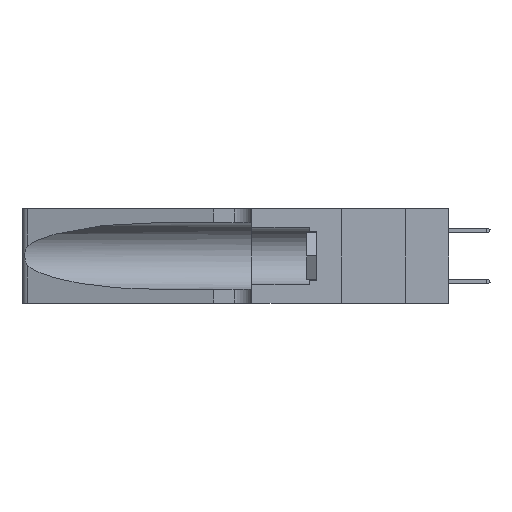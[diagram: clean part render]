
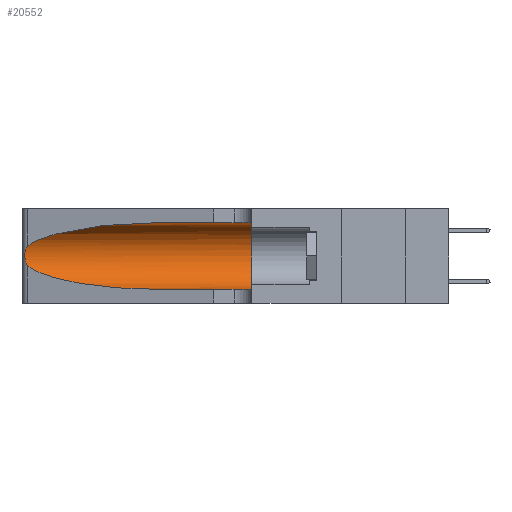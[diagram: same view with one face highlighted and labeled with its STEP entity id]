
A CAD part, left-side view. The second image highlights one B-rep face of the part: STEP entity #20552.
In plain terms, the highlighted cylindrical face has radius 3.308 mm (diameter 6.617 mm), a partial arc.
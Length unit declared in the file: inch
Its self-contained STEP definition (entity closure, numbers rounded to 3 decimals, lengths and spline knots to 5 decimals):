
#764 = EDGE_CURVE ( 'NONE', #38939, #9621, #17891, .T. ) ;
#1037 = CARTESIAN_POINT ( 'NONE',  ( 0.25487, 1.22718, 0.22369 ) ) ;
#1170 = CARTESIAN_POINT ( 'NONE',  ( 0.26075, 1.23896, 0.19203 ) ) ;
#2813 =( BOUNDED_CURVE ( )  B_SPLINE_CURVE ( 3, ( #10790, #7544, #30076, #33336 ),
 .UNSPECIFIED., .F., .F. ) 
 B_SPLINE_CURVE_WITH_KNOTS ( ( 4, 4 ),
 ( 1.5708, 2.84003 ),
 .UNSPECIFIED. ) 
 CURVE ( )  GEOMETRIC_REPRESENTATION_ITEM ( )  RATIONAL_B_SPLINE_CURVE ( ( 1., 0.87, 0.87, 1. ) ) 
 REPRESENTATION_ITEM ( '' )  );
#4483 = CARTESIAN_POINT ( 'NONE',  ( 0.26017, 1.23833, 0.17102 ) ) ;
#5992 = ORIENTED_EDGE ( 'NONE', *, *, #22381, .F. ) ;
#6490 = CARTESIAN_POINT ( 'NONE',  ( 0.25487, 1.22718, 0.14631 ) ) ;
#6668 = EDGE_CURVE ( 'NONE', #27552, #9397, #2813, .T. ) ;
#7430 = CARTESIAN_POINT ( 'NONE',  ( 0.1305, 1.61858, 0.05475 ) ) ;
#7544 = CARTESIAN_POINT ( 'NONE',  ( 0.18966, 0.96281, 0.31525 ) ) ;
#7632 = CARTESIAN_POINT ( 'NONE',  ( 0.25555, 1.22994, 0.2215 ) ) ;
#7770 = CARTESIAN_POINT ( 'NONE',  ( 0.25789, 1.23486, 0.15765 ) ) ;
#8104 = CYLINDRICAL_SURFACE ( 'NONE', #29977, 0.13025 ) ;
#8883 = CARTESIAN_POINT ( 'NONE',  ( 0.1305, 0.35, 0.05475 ) ) ;
#9397 = VERTEX_POINT ( 'NONE', #16761 ) ;
#9621 = VERTEX_POINT ( 'NONE', #17866 ) ;
#10143 = FACE_OUTER_BOUND ( 'NONE', #13462, .T. ) ;
#10790 = CARTESIAN_POINT ( 'NONE',  ( 0.1305, 0.72297, 0.31525 ) ) ;
#11026 = CARTESIAN_POINT ( 'NONE',  ( 0.25555, 1.22993, 0.14849 ) ) ;
#11373 = ORIENTED_EDGE ( 'NONE', *, *, #764, .T. ) ;
#11673 = B_SPLINE_CURVE_WITH_KNOTS ( 'NONE', 3,
 ( #1037, #7632, #36651, #17365, #39866, #20601, #1170, #23839, #4483, #27059, #7770, #30301, #11026, #33558 ),
 .UNSPECIFIED., .F., .F.,
 ( 4, 2, 2, 2, 2, 2, 4 ),
 ( 0., 0.00027, 0.00053, 0.00107, 0.0016, 0.00187, 0.00214 ),
 .UNSPECIFIED. ) ;
#12667 = CARTESIAN_POINT ( 'NONE',  ( 0.1305, 1.61858, 0.185 ) ) ;
#13123 = CARTESIAN_POINT ( 'NONE',  ( 0.1305, 0.35, 0.185 ) ) ;
#13462 = EDGE_LOOP ( 'NONE', ( #30935, #40917, #11373, #40772, #5992, #27935 ) ) ;
#14222 = CARTESIAN_POINT ( 'NONE',  ( 0.2373, 1.15595, 0.08982 ) ) ;
#15902 = DIRECTION ( 'NONE',  ( 0., 0., -1. ) ) ;
#16385 = DIRECTION ( 'NONE',  ( 0., 0., 1. ) ) ;
#16761 = CARTESIAN_POINT ( 'NONE',  ( 0.25487, 1.22718, 0.22369 ) ) ;
#17365 = CARTESIAN_POINT ( 'NONE',  ( 0.25787, 1.23484, 0.2124 ) ) ;
#17489 = CARTESIAN_POINT ( 'NONE',  ( 0.1305, 0.72297, 0.05475 ) ) ;
#17866 = CARTESIAN_POINT ( 'NONE',  ( 0.1305, 0.72297, 0.05475 ) ) ;
#17891 =( BOUNDED_CURVE ( )  B_SPLINE_CURVE ( 3, ( #27045, #14222, #33543, #17489 ),
 .UNSPECIFIED., .F., .T. ) 
 B_SPLINE_CURVE_WITH_KNOTS ( ( 4, 4 ),
 ( 3.44316, 4.71239 ),
 .UNSPECIFIED. ) 
 CURVE ( )  GEOMETRIC_REPRESENTATION_ITEM ( )  RATIONAL_B_SPLINE_CURVE ( ( 1., 0.87, 0.87, 1. ) ) 
 REPRESENTATION_ITEM ( '' )  );
#18500 = CARTESIAN_POINT ( 'NONE',  ( 0.1305, 1.61858, 0.31525 ) ) ;
#19643 = LINE ( 'NONE', #18500, #35775 ) ;
#20552 = ADVANCED_FACE ( 'NONE', ( #10143 ), #8104, .F. ) ;
#20601 = CARTESIAN_POINT ( 'NONE',  ( 0.26018, 1.23835, 0.19895 ) ) ;
#20964 = DIRECTION ( 'NONE',  ( 0., -1., 0. ) ) ;
#21743 = DIRECTION ( 'NONE',  ( 0., -1., 0. ) ) ;
#22381 = EDGE_CURVE ( 'NONE', #29606, #29755, #29484, .T. ) ;
#22907 = LINE ( 'NONE', #7430, #31451 ) ;
#23839 = CARTESIAN_POINT ( 'NONE',  ( 0.26075, 1.23896, 0.178 ) ) ;
#25471 = DIRECTION ( 'NONE',  ( 0., -1., 0. ) ) ;
#25508 = EDGE_CURVE ( 'NONE', #27552, #29606, #19643, .T. ) ;
#27045 = CARTESIAN_POINT ( 'NONE',  ( 0.25487, 1.22718, 0.14631 ) ) ;
#27059 = CARTESIAN_POINT ( 'NONE',  ( 0.25856, 1.23593, 0.16098 ) ) ;
#27552 = VERTEX_POINT ( 'NONE', #33413 ) ;
#27935 = ORIENTED_EDGE ( 'NONE', *, *, #25508, .F. ) ;
#29484 = CIRCLE ( 'NONE', #39481, 0.13025 ) ;
#29606 = VERTEX_POINT ( 'NONE', #33825 ) ;
#29755 = VERTEX_POINT ( 'NONE', #8883 ) ;
#29977 = AXIS2_PLACEMENT_3D ( 'NONE', #12667, #25471, #15902 ) ;
#30076 = CARTESIAN_POINT ( 'NONE',  ( 0.2373, 1.15595, 0.28018 ) ) ;
#30301 = CARTESIAN_POINT ( 'NONE',  ( 0.25639, 1.23186, 0.15144 ) ) ;
#30554 = EDGE_CURVE ( 'NONE', #9621, #29755, #22907, .T. ) ;
#30935 = ORIENTED_EDGE ( 'NONE', *, *, #6668, .T. ) ;
#31451 = VECTOR ( 'NONE', #20964, 39.37008 ) ;
#33336 = CARTESIAN_POINT ( 'NONE',  ( 0.25487, 1.22718, 0.22369 ) ) ;
#33413 = CARTESIAN_POINT ( 'NONE',  ( 0.1305, 0.72297, 0.31525 ) ) ;
#33543 = CARTESIAN_POINT ( 'NONE',  ( 0.18966, 0.96281, 0.05475 ) ) ;
#33558 = CARTESIAN_POINT ( 'NONE',  ( 0.25487, 1.22718, 0.14631 ) ) ;
#33825 = CARTESIAN_POINT ( 'NONE',  ( 0.1305, 0.35, 0.31525 ) ) ;
#35672 = DIRECTION ( 'NONE',  ( 0., 1., 0. ) ) ;
#35775 = VECTOR ( 'NONE', #21743, 39.37008 ) ;
#36651 = CARTESIAN_POINT ( 'NONE',  ( 0.25639, 1.23184, 0.21858 ) ) ;
#38939 = VERTEX_POINT ( 'NONE', #6490 ) ;
#39481 = AXIS2_PLACEMENT_3D ( 'NONE', #13123, #35672, #16385 ) ;
#39866 = CARTESIAN_POINT ( 'NONE',  ( 0.25854, 1.2359, 0.20912 ) ) ;
#40772 = ORIENTED_EDGE ( 'NONE', *, *, #30554, .T. ) ;
#40816 = EDGE_CURVE ( 'NONE', #9397, #38939, #11673, .T. ) ;
#40917 = ORIENTED_EDGE ( 'NONE', *, *, #40816, .T. ) ;
